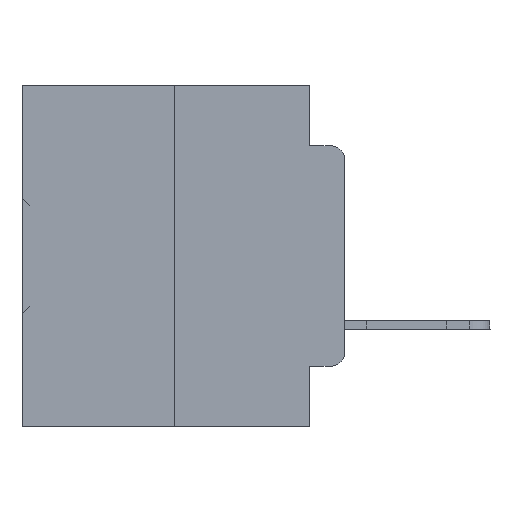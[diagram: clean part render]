
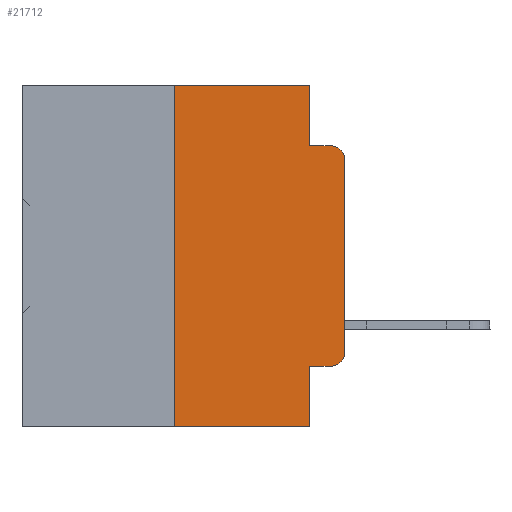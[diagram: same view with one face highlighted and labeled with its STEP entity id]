
A CAD part, left-side view. The second image highlights one B-rep face of the part: STEP entity #21712.
In plain terms, the highlighted planar face has unit normal (-1, 0, 0).
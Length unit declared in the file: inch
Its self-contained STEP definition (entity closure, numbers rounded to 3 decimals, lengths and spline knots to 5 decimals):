
#107 = EDGE_CURVE ( 'NONE', #31464, #11392, #36329, .T. ) ;
#234 = VERTEX_POINT ( 'NONE', #21820 ) ;
#878 = DIRECTION ( 'NONE',  ( 0., 0., -1. ) ) ;
#1322 = CARTESIAN_POINT ( 'NONE',  ( 0., 0.02, -0.3915 ) ) ;
#2700 = VECTOR ( 'NONE', #7084, 39.37008 ) ;
#3057 = DIRECTION ( 'NONE',  ( 0., -1., 0. ) ) ;
#3965 = VECTOR ( 'NONE', #24650, 39.37008 ) ;
#4276 = DIRECTION ( 'NONE',  ( 0., -1., 0. ) ) ;
#4344 = CARTESIAN_POINT ( 'NONE',  ( 0., 0.051, -0.0885 ) ) ;
#4529 = LINE ( 'NONE', #4344, #3965 ) ;
#5970 = ORIENTED_EDGE ( 'NONE', *, *, #15092, .T. ) ;
#6387 = DIRECTION ( 'NONE',  ( 1., 0., 0. ) ) ;
#7059 = VECTOR ( 'NONE', #21859, 39.37008 ) ;
#7084 = DIRECTION ( 'NONE',  ( 0., 0., 1. ) ) ;
#7740 = LINE ( 'NONE', #15732, #33145 ) ;
#8306 = LINE ( 'NONE', #13832, #36664 ) ;
#8326 = EDGE_CURVE ( 'NONE', #34135, #26236, #4529, .T. ) ;
#8889 = VERTEX_POINT ( 'NONE', #22683 ) ;
#9212 = CIRCLE ( 'NONE', #35912, 0.02 ) ;
#9902 = EDGE_LOOP ( 'NONE', ( #19706, #5970, #20875, #33580, #36649, #22512, #30065, #11845, #26299, #28259 ) ) ;
#10020 = VERTEX_POINT ( 'NONE', #24924 ) ;
#11171 = VECTOR ( 'NONE', #21166, 39.37008 ) ;
#11392 = VERTEX_POINT ( 'NONE', #34608 ) ;
#11436 = EDGE_CURVE ( 'NONE', #11392, #10020, #35922, .T. ) ;
#11845 = ORIENTED_EDGE ( 'NONE', *, *, #13215, .F. ) ;
#13089 = DIRECTION ( 'NONE',  ( 0., 0., -1. ) ) ;
#13186 = LINE ( 'NONE', #19053, #31275 ) ;
#13215 = EDGE_CURVE ( 'NONE', #27025, #234, #32698, .T. ) ;
#13832 = CARTESIAN_POINT ( 'NONE',  ( 0., 0.051, -0.4115 ) ) ;
#14236 = VECTOR ( 'NONE', #3057, 39.37008 ) ;
#15092 = EDGE_CURVE ( 'NONE', #10020, #26236, #9212, .T. ) ;
#15732 = CARTESIAN_POINT ( 'NONE',  ( 0., 0.051, 0. ) ) ;
#18296 = EDGE_CURVE ( 'NONE', #30604, #8889, #25608, .T. ) ;
#18540 = DIRECTION ( 'NONE',  ( 0., 0., -1. ) ) ;
#18776 = DIRECTION ( 'NONE',  ( 0., 0., -1. ) ) ;
#19053 = CARTESIAN_POINT ( 'NONE',  ( 0., 0.473, -0.5 ) ) ;
#19505 = DIRECTION ( 'NONE',  ( 0., -1., 0. ) ) ;
#19706 = ORIENTED_EDGE ( 'NONE', *, *, #11436, .T. ) ;
#20290 = CARTESIAN_POINT ( 'NONE',  ( 0., 0.25, 0. ) ) ;
#20875 = ORIENTED_EDGE ( 'NONE', *, *, #8326, .F. ) ;
#21166 = DIRECTION ( 'NONE',  ( 0., 0., 1. ) ) ;
#21222 = VERTEX_POINT ( 'NONE', #37384 ) ;
#21375 = AXIS2_PLACEMENT_3D ( 'NONE', #35984, #6387, #878 ) ;
#21445 = DIRECTION ( 'NONE',  ( -1., 0., 0. ) ) ;
#21712 = ADVANCED_FACE ( 'NONE', ( #35637 ), #23662, .F. ) ;
#21820 = CARTESIAN_POINT ( 'NONE',  ( 0., 0.051, -0.5 ) ) ;
#21859 = DIRECTION ( 'NONE',  ( 0., 0., -1. ) ) ;
#22512 = ORIENTED_EDGE ( 'NONE', *, *, #30046, .F. ) ;
#22683 = CARTESIAN_POINT ( 'NONE',  ( 0., 0.051, 0. ) ) ;
#23662 = PLANE ( 'NONE',  #21375 ) ;
#24000 = LINE ( 'NONE', #35596, #11171 ) ;
#24650 = DIRECTION ( 'NONE',  ( 0., -1., 0. ) ) ;
#24924 = CARTESIAN_POINT ( 'NONE',  ( 0., 0., -0.1085 ) ) ;
#25457 = EDGE_CURVE ( 'NONE', #27025, #31464, #8306, .T. ) ;
#25608 = LINE ( 'NONE', #28484, #14236 ) ;
#26236 = VERTEX_POINT ( 'NONE', #36589 ) ;
#26299 = ORIENTED_EDGE ( 'NONE', *, *, #25457, .T. ) ;
#27025 = VERTEX_POINT ( 'NONE', #32356 ) ;
#27258 = DIRECTION ( 'NONE',  ( -1., 0., 0. ) ) ;
#27977 = CARTESIAN_POINT ( 'NONE',  ( 0., 0.051, -0.0885 ) ) ;
#28259 = ORIENTED_EDGE ( 'NONE', *, *, #107, .T. ) ;
#28484 = CARTESIAN_POINT ( 'NONE',  ( 0., 0.473, 0. ) ) ;
#29921 = CARTESIAN_POINT ( 'NONE',  ( 0., 0.02, -0.1085 ) ) ;
#30046 = EDGE_CURVE ( 'NONE', #21222, #30604, #24000, .T. ) ;
#30065 = ORIENTED_EDGE ( 'NONE', *, *, #33284, .T. ) ;
#30604 = VERTEX_POINT ( 'NONE', #20290 ) ;
#31275 = VECTOR ( 'NONE', #4276, 39.37008 ) ;
#31464 = VERTEX_POINT ( 'NONE', #35483 ) ;
#32356 = CARTESIAN_POINT ( 'NONE',  ( 0., 0.051, -0.4115 ) ) ;
#32698 = LINE ( 'NONE', #36302, #7059 ) ;
#33145 = VECTOR ( 'NONE', #18776, 39.37008 ) ;
#33284 = EDGE_CURVE ( 'NONE', #21222, #234, #13186, .T. ) ;
#33580 = ORIENTED_EDGE ( 'NONE', *, *, #35372, .F. ) ;
#34135 = VERTEX_POINT ( 'NONE', #27977 ) ;
#34608 = CARTESIAN_POINT ( 'NONE',  ( 0., 0., -0.3915 ) ) ;
#35372 = EDGE_CURVE ( 'NONE', #8889, #34135, #7740, .T. ) ;
#35483 = CARTESIAN_POINT ( 'NONE',  ( 0., 0.02, -0.4115 ) ) ;
#35596 = CARTESIAN_POINT ( 'NONE',  ( 0., 0.25, 0. ) ) ;
#35637 = FACE_OUTER_BOUND ( 'NONE', #9902, .T. ) ;
#35912 = AXIS2_PLACEMENT_3D ( 'NONE', #29921, #27258, #18540 ) ;
#35922 = LINE ( 'NONE', #36116, #2700 ) ;
#35984 = CARTESIAN_POINT ( 'NONE',  ( 0., 0.473, 0. ) ) ;
#36116 = CARTESIAN_POINT ( 'NONE',  ( 0., 0., 0. ) ) ;
#36302 = CARTESIAN_POINT ( 'NONE',  ( 0., 0.051, 0. ) ) ;
#36329 = CIRCLE ( 'NONE', #36935, 0.02 ) ;
#36589 = CARTESIAN_POINT ( 'NONE',  ( 0., 0.02, -0.0885 ) ) ;
#36649 = ORIENTED_EDGE ( 'NONE', *, *, #18296, .F. ) ;
#36664 = VECTOR ( 'NONE', #19505, 39.37008 ) ;
#36935 = AXIS2_PLACEMENT_3D ( 'NONE', #1322, #21445, #13089 ) ;
#37384 = CARTESIAN_POINT ( 'NONE',  ( 0., 0.25, -0.5 ) ) ;
